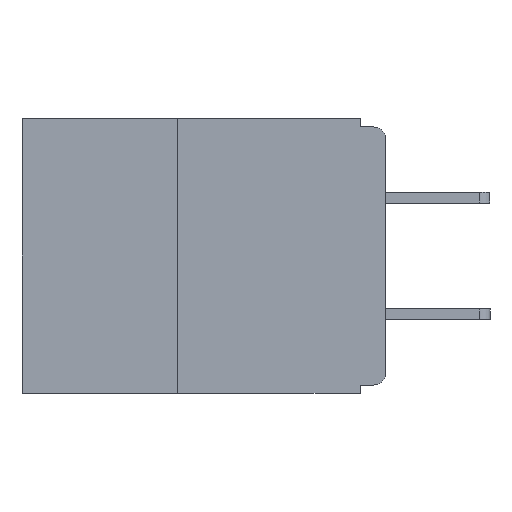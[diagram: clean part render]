
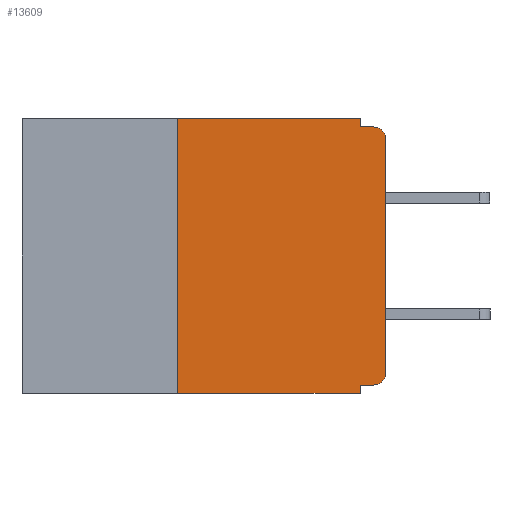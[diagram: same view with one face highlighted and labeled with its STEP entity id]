
A CAD part, left-side view. The second image highlights one B-rep face of the part: STEP entity #13609.
In plain terms, the highlighted planar face has unit normal (-1, 0, 0).
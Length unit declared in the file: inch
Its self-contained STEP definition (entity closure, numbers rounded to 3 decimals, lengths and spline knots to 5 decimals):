
#676 = AXIS2_PLACEMENT_3D ( 'NONE', #18906, #6383, #21119 ) ;
#861 = CARTESIAN_POINT ( 'NONE',  ( 0., 0.25, -0.33 ) ) ;
#1968 = DIRECTION ( 'NONE',  ( 0., 0., -1. ) ) ;
#2165 = DIRECTION ( 'NONE',  ( 0., -1., 0. ) ) ;
#3592 = CARTESIAN_POINT ( 'NONE',  ( 0., 0.031, -0.33 ) ) ;
#4317 = VECTOR ( 'NONE', #19935, 39.37008 ) ;
#4381 = EDGE_CURVE ( 'NONE', #15185, #24145, #16136, .T. ) ;
#4485 = VERTEX_POINT ( 'NONE', #4808 ) ;
#4808 = CARTESIAN_POINT ( 'NONE',  ( 0., 0.015, -0.01 ) ) ;
#5001 = VECTOR ( 'NONE', #25160, 39.37008 ) ;
#5106 = ORIENTED_EDGE ( 'NONE', *, *, #16657, .T. ) ;
#5535 = VECTOR ( 'NONE', #24511, 39.37008 ) ;
#5546 = CARTESIAN_POINT ( 'NONE',  ( 0., 0.031, 0. ) ) ;
#5621 = VERTEX_POINT ( 'NONE', #9922 ) ;
#6383 = DIRECTION ( 'NONE',  ( -1., 0., 0. ) ) ;
#6474 = DIRECTION ( 'NONE',  ( 0., 1., 0. ) ) ;
#6797 = CARTESIAN_POINT ( 'NONE',  ( 0., 0., -0.305 ) ) ;
#6851 = CARTESIAN_POINT ( 'NONE',  ( 0., 0., -0.32 ) ) ;
#7062 = LINE ( 'NONE', #20179, #11925 ) ;
#8368 = CARTESIAN_POINT ( 'NONE',  ( 0., 0.25, 0. ) ) ;
#9317 = EDGE_CURVE ( 'NONE', #21215, #16694, #10036, .T. ) ;
#9751 = EDGE_CURVE ( 'NONE', #24145, #5621, #21670, .T. ) ;
#9922 = CARTESIAN_POINT ( 'NONE',  ( 0., 0.031, -0.33 ) ) ;
#9953 = DIRECTION ( 'NONE',  ( -1., 0., 0. ) ) ;
#10006 = VECTOR ( 'NONE', #6474, 39.37008 ) ;
#10036 = LINE ( 'NONE', #12514, #26158 ) ;
#10267 = CARTESIAN_POINT ( 'NONE',  ( 0., 0.437, 0. ) ) ;
#10327 = CIRCLE ( 'NONE', #27002, 0.015 ) ;
#10563 = EDGE_CURVE ( 'NONE', #15185, #21215, #10327, .T. ) ;
#11422 = AXIS2_PLACEMENT_3D ( 'NONE', #10267, #14402, #1968 ) ;
#11425 = CARTESIAN_POINT ( 'NONE',  ( 0., 0., -0.01 ) ) ;
#11695 = ORIENTED_EDGE ( 'NONE', *, *, #11791, .F. ) ;
#11791 = EDGE_CURVE ( 'NONE', #15437, #17076, #7062, .T. ) ;
#11925 = VECTOR ( 'NONE', #15838, 39.37008 ) ;
#12346 = PLANE ( 'NONE',  #11422 ) ;
#12505 = CARTESIAN_POINT ( 'NONE',  ( 0., 0.25, -0.33 ) ) ;
#12514 = CARTESIAN_POINT ( 'NONE',  ( 0., 0., 0. ) ) ;
#12993 = CARTESIAN_POINT ( 'NONE',  ( 0., 0.031, -0.01 ) ) ;
#13566 = VECTOR ( 'NONE', #26161, 39.37008 ) ;
#13609 = ADVANCED_FACE ( 'NONE', ( #19779 ), #12346, .F. ) ;
#14402 = DIRECTION ( 'NONE',  ( 1., 0., 0. ) ) ;
#14447 = EDGE_CURVE ( 'NONE', #26128, #4485, #15288, .T. ) ;
#14919 = VECTOR ( 'NONE', #2165, 39.37008 ) ;
#15026 = CARTESIAN_POINT ( 'NONE',  ( 0., 0.031, -0.32 ) ) ;
#15185 = VERTEX_POINT ( 'NONE', #22312 ) ;
#15288 = LINE ( 'NONE', #11425, #4317 ) ;
#15437 = VERTEX_POINT ( 'NONE', #8368 ) ;
#15838 = DIRECTION ( 'NONE',  ( 0., -1., 0. ) ) ;
#16136 = LINE ( 'NONE', #6851, #10006 ) ;
#16188 = ORIENTED_EDGE ( 'NONE', *, *, #9751, .F. ) ;
#16657 = EDGE_CURVE ( 'NONE', #24301, #5621, #20031, .T. ) ;
#16694 = VERTEX_POINT ( 'NONE', #21226 ) ;
#16697 = CARTESIAN_POINT ( 'NONE',  ( 0., 0.437, -0.33 ) ) ;
#17076 = VERTEX_POINT ( 'NONE', #5546 ) ;
#17170 = CIRCLE ( 'NONE', #676, 0.015 ) ;
#18827 = EDGE_CURVE ( 'NONE', #17076, #26128, #19948, .T. ) ;
#18906 = CARTESIAN_POINT ( 'NONE',  ( 0., 0.015, -0.025 ) ) ;
#19779 = FACE_OUTER_BOUND ( 'NONE', #26919, .T. ) ;
#19935 = DIRECTION ( 'NONE',  ( 0., -1., 0. ) ) ;
#19948 = LINE ( 'NONE', #22112, #13566 ) ;
#20031 = LINE ( 'NONE', #16697, #14919 ) ;
#20179 = CARTESIAN_POINT ( 'NONE',  ( 0., 0.437, 0. ) ) ;
#20755 = ORIENTED_EDGE ( 'NONE', *, *, #9317, .T. ) ;
#21119 = DIRECTION ( 'NONE',  ( 0., 0., -1. ) ) ;
#21215 = VERTEX_POINT ( 'NONE', #6797 ) ;
#21226 = CARTESIAN_POINT ( 'NONE',  ( 0., 0., -0.025 ) ) ;
#21383 = ORIENTED_EDGE ( 'NONE', *, *, #10563, .T. ) ;
#21670 = LINE ( 'NONE', #3592, #5535 ) ;
#21845 = ORIENTED_EDGE ( 'NONE', *, *, #25337, .T. ) ;
#22009 = ORIENTED_EDGE ( 'NONE', *, *, #22785, .F. ) ;
#22112 = CARTESIAN_POINT ( 'NONE',  ( 0., 0.031, 0. ) ) ;
#22312 = CARTESIAN_POINT ( 'NONE',  ( 0., 0.015, -0.32 ) ) ;
#22337 = ORIENTED_EDGE ( 'NONE', *, *, #14447, .F. ) ;
#22623 = CARTESIAN_POINT ( 'NONE',  ( 0., 0.015, -0.305 ) ) ;
#22785 = EDGE_CURVE ( 'NONE', #24301, #15437, #26591, .T. ) ;
#23463 = ORIENTED_EDGE ( 'NONE', *, *, #18827, .F. ) ;
#24145 = VERTEX_POINT ( 'NONE', #15026 ) ;
#24293 = ORIENTED_EDGE ( 'NONE', *, *, #4381, .F. ) ;
#24301 = VERTEX_POINT ( 'NONE', #861 ) ;
#24511 = DIRECTION ( 'NONE',  ( 0., 0., -1. ) ) ;
#24700 = DIRECTION ( 'NONE',  ( 0., 0., -1. ) ) ;
#25160 = DIRECTION ( 'NONE',  ( 0., 0., 1. ) ) ;
#25174 = DIRECTION ( 'NONE',  ( 0., 0., 1. ) ) ;
#25337 = EDGE_CURVE ( 'NONE', #16694, #4485, #17170, .T. ) ;
#26128 = VERTEX_POINT ( 'NONE', #12993 ) ;
#26158 = VECTOR ( 'NONE', #25174, 39.37008 ) ;
#26161 = DIRECTION ( 'NONE',  ( 0., 0., -1. ) ) ;
#26591 = LINE ( 'NONE', #12505, #5001 ) ;
#26919 = EDGE_LOOP ( 'NONE', ( #20755, #21845, #22337, #23463, #11695, #22009, #5106, #16188, #24293, #21383 ) ) ;
#27002 = AXIS2_PLACEMENT_3D ( 'NONE', #22623, #9953, #24700 ) ;
